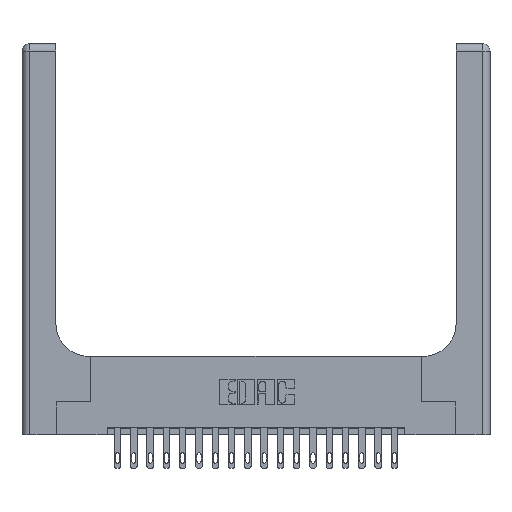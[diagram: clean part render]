
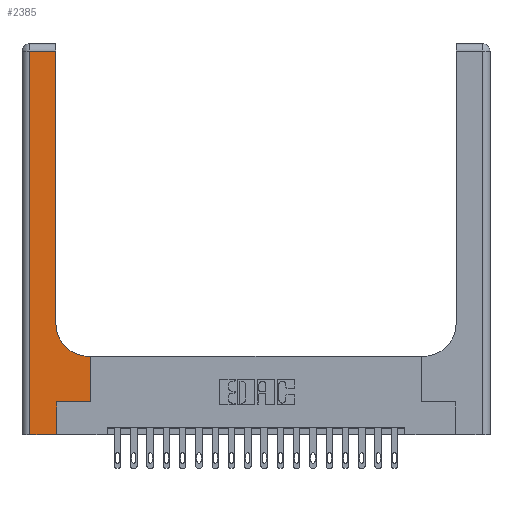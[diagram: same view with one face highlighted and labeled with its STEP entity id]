
A CAD part, top view. The second image highlights one B-rep face of the part: STEP entity #2385.
In plain terms, the highlighted planar face has unit normal (0, 0, 1).
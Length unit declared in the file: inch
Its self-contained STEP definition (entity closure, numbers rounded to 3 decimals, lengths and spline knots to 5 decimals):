
#16 = VECTOR ( 'NONE', #17310, 39.37008 ) ;
#18 = CARTESIAN_POINT ( 'NONE',  ( 0.528, 0.6, 0.37 ) ) ;
#144 = DIRECTION ( 'NONE',  ( 0., 1., 0. ) ) ;
#164 = ORIENTED_EDGE ( 'NONE', *, *, #18326, .T. ) ;
#185 = ORIENTED_EDGE ( 'NONE', *, *, #18954, .T. ) ;
#202 = VERTEX_POINT ( 'NONE', #5935 ) ;
#751 = CARTESIAN_POINT ( 'NONE',  ( 0.06, 3., 0.37 ) ) ;
#1572 = VERTEX_POINT ( 'NONE', #20095 ) ;
#1972 = DIRECTION ( 'NONE',  ( -1., 0., 0. ) ) ;
#2089 = EDGE_CURVE ( 'NONE', #14021, #202, #3807, .T. ) ;
#2247 = DIRECTION ( 'NONE',  ( 1., 0., 0. ) ) ;
#2385 = ADVANCED_FACE ( 'NONE', ( #4528 ), #7756, .F. ) ;
#2406 = EDGE_CURVE ( 'NONE', #12987, #6744, #7657, .T. ) ;
#2509 = LINE ( 'NONE', #10629, #7555 ) ;
#2583 = VECTOR ( 'NONE', #8332, 39.37008 ) ;
#2629 = CARTESIAN_POINT ( 'NONE',  ( 0.06, 0., 0.37 ) ) ;
#3278 = VECTOR ( 'NONE', #4336, 39.37008 ) ;
#3725 = VERTEX_POINT ( 'NONE', #11681 ) ;
#3807 = LINE ( 'NONE', #14527, #10628 ) ;
#4101 = CARTESIAN_POINT ( 'NONE',  ( 0.26, 0.85, 0.37 ) ) ;
#4264 = EDGE_CURVE ( 'NONE', #6744, #1572, #5093, .T. ) ;
#4336 = DIRECTION ( 'NONE',  ( 1., 0., 0. ) ) ;
#4480 = DIRECTION ( 'NONE',  ( -1., 0., 0. ) ) ;
#4528 = FACE_OUTER_BOUND ( 'NONE', #10107, .T. ) ;
#5093 = LINE ( 'NONE', #8111, #15993 ) ;
#5446 = EDGE_CURVE ( 'NONE', #9702, #10512, #13938, .T. ) ;
#5935 = CARTESIAN_POINT ( 'NONE',  ( 0.265, 0., 0.37 ) ) ;
#6301 = EDGE_CURVE ( 'NONE', #19257, #12987, #6429, .T. ) ;
#6429 = CIRCLE ( 'NONE', #7087, 0.25 ) ;
#6744 = VERTEX_POINT ( 'NONE', #9147 ) ;
#6872 = LINE ( 'NONE', #751, #2583 ) ;
#7087 = AXIS2_PLACEMENT_3D ( 'NONE', #15749, #20531, #13778 ) ;
#7555 = VECTOR ( 'NONE', #4480, 39.37008 ) ;
#7657 = LINE ( 'NONE', #17409, #16 ) ;
#7701 = ORIENTED_EDGE ( 'NONE', *, *, #2406, .T. ) ;
#7756 = PLANE ( 'NONE',  #10987 ) ;
#8044 = VECTOR ( 'NONE', #12683, 39.37008 ) ;
#8111 = CARTESIAN_POINT ( 'NONE',  ( 0., 2.94, 0.37 ) ) ;
#8232 = LINE ( 'NONE', #12921, #14544 ) ;
#8332 = DIRECTION ( 'NONE',  ( 0., -1., 0. ) ) ;
#9127 = CARTESIAN_POINT ( 'NONE',  ( 0.265, 0.25, 0.37 ) ) ;
#9147 = CARTESIAN_POINT ( 'NONE',  ( 0.26, 2.94, 0.37 ) ) ;
#9171 = CARTESIAN_POINT ( 'NONE',  ( 0.51, 0.6, 0.37 ) ) ;
#9325 = CARTESIAN_POINT ( 'NONE',  ( 0., 3., 0.37 ) ) ;
#9702 = VERTEX_POINT ( 'NONE', #16325 ) ;
#9973 = ORIENTED_EDGE ( 'NONE', *, *, #20127, .T. ) ;
#10107 = EDGE_LOOP ( 'NONE', ( #7701, #18786, #18302, #18663, #185, #9973, #17605, #164, #14045 ) ) ;
#10512 = VERTEX_POINT ( 'NONE', #18 ) ;
#10628 = VECTOR ( 'NONE', #2247, 39.37008 ) ;
#10629 = CARTESIAN_POINT ( 'NONE',  ( 0.26, 0.6, 0.37 ) ) ;
#10987 = AXIS2_PLACEMENT_3D ( 'NONE', #9325, #11088, #15661 ) ;
#11088 = DIRECTION ( 'NONE',  ( 0., 0., -1. ) ) ;
#11681 = CARTESIAN_POINT ( 'NONE',  ( 0.265, 0.25, 0.37 ) ) ;
#12146 = LINE ( 'NONE', #9127, #3278 ) ;
#12683 = DIRECTION ( 'NONE',  ( 0., 1., 0. ) ) ;
#12921 = CARTESIAN_POINT ( 'NONE',  ( 0.265, 0., 0.37 ) ) ;
#12987 = VERTEX_POINT ( 'NONE', #4101 ) ;
#13778 = DIRECTION ( 'NONE',  ( 1., 0., 0. ) ) ;
#13938 = LINE ( 'NONE', #17557, #8044 ) ;
#14021 = VERTEX_POINT ( 'NONE', #2629 ) ;
#14045 = ORIENTED_EDGE ( 'NONE', *, *, #6301, .T. ) ;
#14527 = CARTESIAN_POINT ( 'NONE',  ( 0., 0., 0.37 ) ) ;
#14544 = VECTOR ( 'NONE', #144, 39.37008 ) ;
#15661 = DIRECTION ( 'NONE',  ( -1., 0., 0. ) ) ;
#15749 = CARTESIAN_POINT ( 'NONE',  ( 0.51, 0.85, 0.37 ) ) ;
#15993 = VECTOR ( 'NONE', #1972, 39.37008 ) ;
#16325 = CARTESIAN_POINT ( 'NONE',  ( 0.528, 0.25, 0.37 ) ) ;
#17310 = DIRECTION ( 'NONE',  ( 0., 1., 0. ) ) ;
#17409 = CARTESIAN_POINT ( 'NONE',  ( 0.26, 3., 0.37 ) ) ;
#17557 = CARTESIAN_POINT ( 'NONE',  ( 0.528, 0.25, 0.37 ) ) ;
#17605 = ORIENTED_EDGE ( 'NONE', *, *, #5446, .T. ) ;
#18149 = EDGE_CURVE ( 'NONE', #1572, #14021, #6872, .T. ) ;
#18302 = ORIENTED_EDGE ( 'NONE', *, *, #18149, .T. ) ;
#18326 = EDGE_CURVE ( 'NONE', #10512, #19257, #2509, .T. ) ;
#18663 = ORIENTED_EDGE ( 'NONE', *, *, #2089, .T. ) ;
#18786 = ORIENTED_EDGE ( 'NONE', *, *, #4264, .T. ) ;
#18954 = EDGE_CURVE ( 'NONE', #202, #3725, #8232, .T. ) ;
#19257 = VERTEX_POINT ( 'NONE', #9171 ) ;
#20095 = CARTESIAN_POINT ( 'NONE',  ( 0.06, 2.94, 0.37 ) ) ;
#20127 = EDGE_CURVE ( 'NONE', #3725, #9702, #12146, .T. ) ;
#20531 = DIRECTION ( 'NONE',  ( 0., 0., -1. ) ) ;
